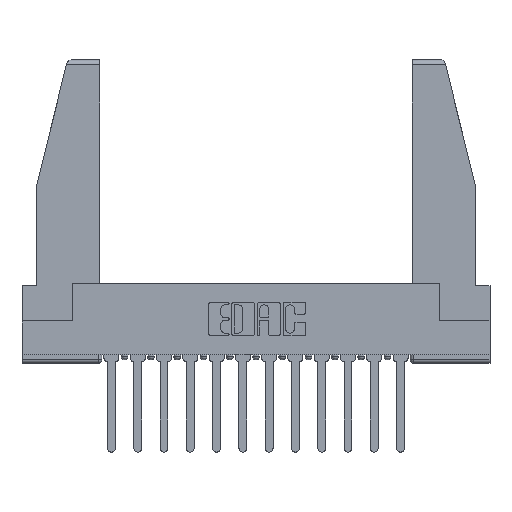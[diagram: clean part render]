
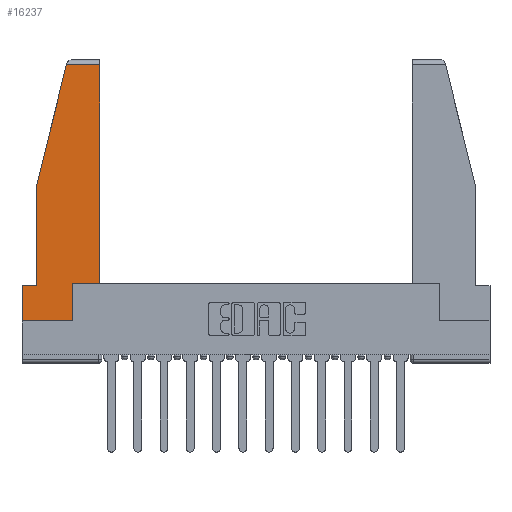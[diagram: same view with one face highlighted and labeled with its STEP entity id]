
A CAD part, top view. The second image highlights one B-rep face of the part: STEP entity #16237.
In plain terms, the highlighted planar face has unit normal (0, 0, 1).
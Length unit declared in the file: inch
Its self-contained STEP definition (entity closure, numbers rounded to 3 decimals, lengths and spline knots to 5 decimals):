
#337 = CARTESIAN_POINT ( 'NONE',  ( 0., 1.52, 0. ) ) ;
#424 = EDGE_CURVE ( 'NONE', #13435, #437, #10921, .T. ) ;
#437 = VERTEX_POINT ( 'NONE', #10138 ) ;
#680 = VERTEX_POINT ( 'NONE', #7885 ) ;
#923 = CARTESIAN_POINT ( 'NONE',  ( 0., 0., 0. ) ) ;
#952 = CARTESIAN_POINT ( 'NONE',  ( 0.461, 0.223, 0. ) ) ;
#1082 = DIRECTION ( 'NONE',  ( 1., 0., 0. ) ) ;
#2012 = LINE ( 'NONE', #952, #9978 ) ;
#2108 = EDGE_LOOP ( 'NONE', ( #6025, #6857, #3612, #15012, #14305, #2324, #4011, #15340, #11002 ) ) ;
#2324 = ORIENTED_EDGE ( 'NONE', *, *, #11059, .T. ) ;
#2355 = DIRECTION ( 'NONE',  ( 0., 0., 1. ) ) ;
#2765 = DIRECTION ( 'NONE',  ( 0., -1., 0. ) ) ;
#2876 = LINE ( 'NONE', #9113, #12584 ) ;
#2998 = CARTESIAN_POINT ( 'NONE',  ( 0.297, 0., 0. ) ) ;
#3225 = LINE ( 'NONE', #9132, #10004 ) ;
#3259 = LINE ( 'NONE', #7168, #12571 ) ;
#3428 = DIRECTION ( 'NONE',  ( 0., 1., 0. ) ) ;
#3606 = VERTEX_POINT ( 'NONE', #13988 ) ;
#3612 = ORIENTED_EDGE ( 'NONE', *, *, #6828, .T. ) ;
#3656 = FACE_OUTER_BOUND ( 'NONE', #2108, .T. ) ;
#3747 = DIRECTION ( 'NONE',  ( 1., 0., 0. ) ) ;
#3824 = DIRECTION ( 'NONE',  ( 0., 1., 0. ) ) ;
#4011 = ORIENTED_EDGE ( 'NONE', *, *, #12361, .T. ) ;
#4803 = DIRECTION ( 'NONE',  ( -0.239, -0.971, 0. ) ) ;
#4989 = CARTESIAN_POINT ( 'NONE',  ( 0.297, 0.223, 0. ) ) ;
#5062 = EDGE_CURVE ( 'NONE', #8380, #680, #8076, .T. ) ;
#5417 = EDGE_CURVE ( 'NONE', #14178, #3606, #2876, .T. ) ;
#5492 = VERTEX_POINT ( 'NONE', #11800 ) ;
#5780 = DIRECTION ( 'NONE',  ( -1., 0., 0. ) ) ;
#6025 = ORIENTED_EDGE ( 'NONE', *, *, #13317, .T. ) ;
#6262 = LINE ( 'NONE', #4989, #15741 ) ;
#6828 = EDGE_CURVE ( 'NONE', #437, #14178, #12366, .T. ) ;
#6857 = ORIENTED_EDGE ( 'NONE', *, *, #424, .T. ) ;
#6962 = CARTESIAN_POINT ( 'NONE',  ( 0.297, 0., 0. ) ) ;
#7168 = CARTESIAN_POINT ( 'NONE',  ( 0., 0.21, 0. ) ) ;
#7496 = CARTESIAN_POINT ( 'NONE',  ( 0.461, 0.223, 0. ) ) ;
#7885 = CARTESIAN_POINT ( 'NONE',  ( 0.297, 0.223, 0. ) ) ;
#8076 = LINE ( 'NONE', #2998, #8669 ) ;
#8380 = VERTEX_POINT ( 'NONE', #6962 ) ;
#8669 = VECTOR ( 'NONE', #3428, 39.37008 ) ;
#8708 = PLANE ( 'NONE',  #13265 ) ;
#9113 = CARTESIAN_POINT ( 'NONE',  ( 0.086, 0.8, 0. ) ) ;
#9132 = CARTESIAN_POINT ( 'NONE',  ( 0., 0., 0. ) ) ;
#9470 = LINE ( 'NONE', #10907, #9662 ) ;
#9662 = VECTOR ( 'NONE', #5780, 39.37008 ) ;
#9806 = VERTEX_POINT ( 'NONE', #7496 ) ;
#9978 = VECTOR ( 'NONE', #3824, 39.37008 ) ;
#10004 = VECTOR ( 'NONE', #14136, 39.37008 ) ;
#10138 = CARTESIAN_POINT ( 'NONE',  ( 0.2636, 1.52, 0. ) ) ;
#10332 = EDGE_CURVE ( 'NONE', #3606, #14435, #9470, .T. ) ;
#10907 = CARTESIAN_POINT ( 'NONE',  ( 0., 0.21, 0. ) ) ;
#10921 = LINE ( 'NONE', #337, #13476 ) ;
#11002 = ORIENTED_EDGE ( 'NONE', *, *, #15709, .T. ) ;
#11023 = CARTESIAN_POINT ( 'NONE',  ( 0.271, 1.55, 0. ) ) ;
#11059 = EDGE_CURVE ( 'NONE', #14435, #5492, #3259, .T. ) ;
#11129 = CARTESIAN_POINT ( 'NONE',  ( 0., 0.21, 0. ) ) ;
#11578 = VECTOR ( 'NONE', #4803, 39.37008 ) ;
#11800 = CARTESIAN_POINT ( 'NONE',  ( 0., 0., 0. ) ) ;
#12065 = DIRECTION ( 'NONE',  ( -1., 0., 0. ) ) ;
#12361 = EDGE_CURVE ( 'NONE', #5492, #8380, #3225, .T. ) ;
#12366 = LINE ( 'NONE', #11023, #11578 ) ;
#12571 = VECTOR ( 'NONE', #15923, 39.37008 ) ;
#12584 = VECTOR ( 'NONE', #2765, 39.37008 ) ;
#12807 = CARTESIAN_POINT ( 'NONE',  ( 0.461, 1.52, 0. ) ) ;
#13265 = AXIS2_PLACEMENT_3D ( 'NONE', #923, #2355, #1082 ) ;
#13317 = EDGE_CURVE ( 'NONE', #9806, #13435, #2012, .T. ) ;
#13435 = VERTEX_POINT ( 'NONE', #12807 ) ;
#13476 = VECTOR ( 'NONE', #12065, 39.37008 ) ;
#13988 = CARTESIAN_POINT ( 'NONE',  ( 0.086, 0.21, 0. ) ) ;
#14136 = DIRECTION ( 'NONE',  ( 1., 0., 0. ) ) ;
#14159 = CARTESIAN_POINT ( 'NONE',  ( 0.086, 0.8, 0. ) ) ;
#14178 = VERTEX_POINT ( 'NONE', #14159 ) ;
#14305 = ORIENTED_EDGE ( 'NONE', *, *, #10332, .T. ) ;
#14435 = VERTEX_POINT ( 'NONE', #11129 ) ;
#15012 = ORIENTED_EDGE ( 'NONE', *, *, #5417, .T. ) ;
#15340 = ORIENTED_EDGE ( 'NONE', *, *, #5062, .T. ) ;
#15709 = EDGE_CURVE ( 'NONE', #680, #9806, #6262, .T. ) ;
#15741 = VECTOR ( 'NONE', #3747, 39.37008 ) ;
#15923 = DIRECTION ( 'NONE',  ( 0., -1., 0. ) ) ;
#16237 = ADVANCED_FACE ( 'NONE', ( #3656 ), #8708, .T. ) ;
